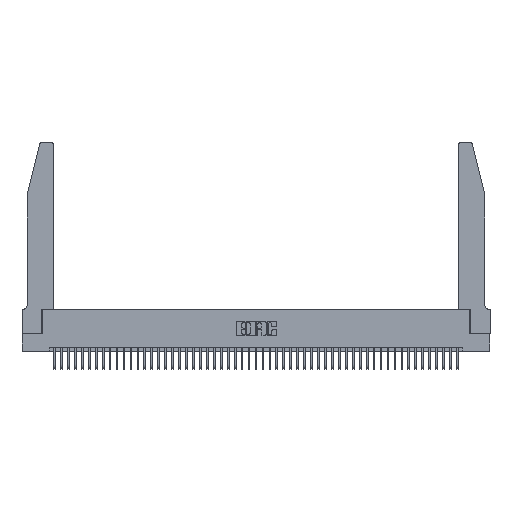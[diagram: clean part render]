
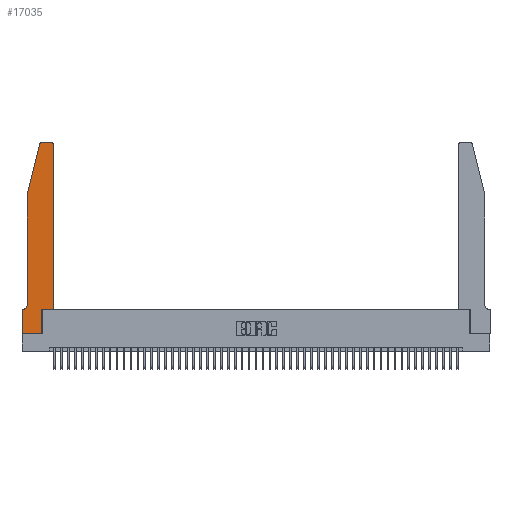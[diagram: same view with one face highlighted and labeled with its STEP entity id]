
A CAD part, top view. The second image highlights one B-rep face of the part: STEP entity #17035.
In plain terms, the highlighted planar face has unit normal (0, 0, 1).
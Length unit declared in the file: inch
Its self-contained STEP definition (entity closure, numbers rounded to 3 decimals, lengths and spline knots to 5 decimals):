
#1237 = AXIS2_PLACEMENT_3D ( 'NONE', #26726, #5091, #30422 ) ;
#1294 = CARTESIAN_POINT ( 'NONE',  ( 0.2865, 0.35, 0.37 ) ) ;
#1839 = FACE_OUTER_BOUND ( 'NONE', #34573, .T. ) ;
#1923 = CARTESIAN_POINT ( 'NONE',  ( 0.4505, 2.72, 0.37 ) ) ;
#2569 = EDGE_CURVE ( 'NONE', #39155, #37777, #5124, .T. ) ;
#3102 = VERTEX_POINT ( 'NONE', #7702 ) ;
#3226 = EDGE_CURVE ( 'NONE', #44333, #39155, #15180, .T. ) ;
#3483 = DIRECTION ( 'NONE',  ( 1., 0., 0. ) ) ;
#3552 = ORIENTED_EDGE ( 'NONE', *, *, #43686, .T. ) ;
#3634 = LINE ( 'NONE', #30653, #21685 ) ;
#3968 = CARTESIAN_POINT ( 'NONE',  ( 0.0755, 2., 0.37 ) ) ;
#4933 = DIRECTION ( 'NONE',  ( 0., 1., 0. ) ) ;
#5091 = DIRECTION ( 'NONE',  ( 0., 0., 1. ) ) ;
#5124 = LINE ( 'NONE', #1294, #23192 ) ;
#5486 = DIRECTION ( 'NONE',  ( 1., 0., 0. ) ) ;
#5744 = CARTESIAN_POINT ( 'NONE',  ( 0.2865, 0.35, 0.37 ) ) ;
#6064 = VERTEX_POINT ( 'NONE', #33162 ) ;
#6067 = VECTOR ( 'NONE', #35936, 39.37008 ) ;
#6370 = VECTOR ( 'NONE', #34168, 39.37008 ) ;
#6822 = VECTOR ( 'NONE', #29985, 39.37008 ) ;
#7702 = CARTESIAN_POINT ( 'NONE',  ( 0.0755, 0.42, 0.37 ) ) ;
#7890 = CARTESIAN_POINT ( 'NONE',  ( 0.284, 2.72, 0.37 ) ) ;
#8151 = LINE ( 'NONE', #14568, #35947 ) ;
#8938 = CIRCLE ( 'NONE', #41493, 0.03 ) ;
#9886 = EDGE_CURVE ( 'NONE', #22141, #3102, #44643, .T. ) ;
#10256 = DIRECTION ( 'NONE',  ( 0., 0., -1. ) ) ;
#11444 = ORIENTED_EDGE ( 'NONE', *, *, #25841, .T. ) ;
#11535 = ORIENTED_EDGE ( 'NONE', *, *, #37563, .T. ) ;
#11543 = DIRECTION ( 'NONE',  ( 1., 0., 0. ) ) ;
#12093 = EDGE_CURVE ( 'NONE', #37777, #46083, #3634, .T. ) ;
#12581 = CARTESIAN_POINT ( 'NONE',  ( 0., 0.35, 0.37 ) ) ;
#14093 = EDGE_CURVE ( 'NONE', #3102, #16471, #29463, .T. ) ;
#14568 = CARTESIAN_POINT ( 'NONE',  ( 0.0755, 2., 0.37 ) ) ;
#14818 = LINE ( 'NONE', #23330, #6370 ) ;
#15180 = LINE ( 'NONE', #41005, #33370 ) ;
#15347 = CARTESIAN_POINT ( 'NONE',  ( 0.4505, 0.35, 0.37 ) ) ;
#15788 = PLANE ( 'NONE',  #1237 ) ;
#16071 = LINE ( 'NONE', #17961, #35427 ) ;
#16227 = VECTOR ( 'NONE', #27158, 39.37008 ) ;
#16444 = VERTEX_POINT ( 'NONE', #30626 ) ;
#16471 = VERTEX_POINT ( 'NONE', #19959 ) ;
#17035 = ADVANCED_FACE ( 'NONE', ( #1839 ), #15788, .T. ) ;
#17961 = CARTESIAN_POINT ( 'NONE',  ( 0.2605, 2.75, 0.37 ) ) ;
#18178 = DIRECTION ( 'NONE',  ( -0.239, -0.971, 0. ) ) ;
#18328 = EDGE_CURVE ( 'NONE', #6064, #42993, #40913, .T. ) ;
#18789 = ORIENTED_EDGE ( 'NONE', *, *, #32397, .T. ) ;
#19389 = ORIENTED_EDGE ( 'NONE', *, *, #2569, .T. ) ;
#19835 = VERTEX_POINT ( 'NONE', #1923 ) ;
#19893 = ORIENTED_EDGE ( 'NONE', *, *, #14093, .T. ) ;
#19959 = CARTESIAN_POINT ( 'NONE',  ( 0.0055, 0.35, 0.37 ) ) ;
#21685 = VECTOR ( 'NONE', #5486, 39.37008 ) ;
#22141 = VERTEX_POINT ( 'NONE', #3968 ) ;
#22804 = CARTESIAN_POINT ( 'NONE',  ( 0.4505, 0.35, 0.37 ) ) ;
#22851 = DIRECTION ( 'NONE',  ( 1., 0., 0. ) ) ;
#23192 = VECTOR ( 'NONE', #4933, 39.37008 ) ;
#23330 = CARTESIAN_POINT ( 'NONE',  ( 0.0755, 0.35, 0.37 ) ) ;
#24068 = EDGE_CURVE ( 'NONE', #19835, #16444, #8938, .T. ) ;
#24372 = ORIENTED_EDGE ( 'NONE', *, *, #35779, .T. ) ;
#25102 = DIRECTION ( 'NONE',  ( 0., 0., 1. ) ) ;
#25841 = EDGE_CURVE ( 'NONE', #16444, #6064, #16071, .T. ) ;
#26061 = LINE ( 'NONE', #15347, #6822 ) ;
#26726 = CARTESIAN_POINT ( 'NONE',  ( 0., 0.35, 0.37 ) ) ;
#27158 = DIRECTION ( 'NONE',  ( 0., -1., 0. ) ) ;
#27617 = AXIS2_PLACEMENT_3D ( 'NONE', #7890, #33242, #11543 ) ;
#28402 = VERTEX_POINT ( 'NONE', #12581 ) ;
#28757 = CARTESIAN_POINT ( 'NONE',  ( 0.0755, 2., 0.37 ) ) ;
#29463 = CIRCLE ( 'NONE', #41853, 0.07 ) ;
#29985 = DIRECTION ( 'NONE',  ( 0., 1., 0. ) ) ;
#30422 = DIRECTION ( 'NONE',  ( 1., 0., 0. ) ) ;
#30626 = CARTESIAN_POINT ( 'NONE',  ( 0.4205, 2.75, 0.37 ) ) ;
#30653 = CARTESIAN_POINT ( 'NONE',  ( 0.4505, 0.35, 0.37 ) ) ;
#31353 = ORIENTED_EDGE ( 'NONE', *, *, #12093, .T. ) ;
#31969 = CARTESIAN_POINT ( 'NONE',  ( 0.0055, 0.42, 0.37 ) ) ;
#32397 = EDGE_CURVE ( 'NONE', #28402, #44333, #44110, .T. ) ;
#33162 = CARTESIAN_POINT ( 'NONE',  ( 0.284, 2.75, 0.37 ) ) ;
#33242 = DIRECTION ( 'NONE',  ( 0., 0., 1. ) ) ;
#33370 = VECTOR ( 'NONE', #22851, 39.37008 ) ;
#33753 = CARTESIAN_POINT ( 'NONE',  ( 0.25487, 2.72718, 0.37 ) ) ;
#34168 = DIRECTION ( 'NONE',  ( -1., 0., 0. ) ) ;
#34358 = CARTESIAN_POINT ( 'NONE',  ( 0., 0., 0.37 ) ) ;
#34573 = EDGE_LOOP ( 'NONE', ( #11444, #39200, #24372, #45470, #19893, #3552, #18789, #35325, #19389, #31353, #11535, #42753 ) ) ;
#35325 = ORIENTED_EDGE ( 'NONE', *, *, #3226, .T. ) ;
#35427 = VECTOR ( 'NONE', #43417, 39.37008 ) ;
#35643 = DIRECTION ( 'NONE',  ( -1., 0., 0. ) ) ;
#35779 = EDGE_CURVE ( 'NONE', #42993, #22141, #8151, .T. ) ;
#35936 = DIRECTION ( 'NONE',  ( 0., -1., 0. ) ) ;
#35947 = VECTOR ( 'NONE', #18178, 39.37008 ) ;
#36103 = CARTESIAN_POINT ( 'NONE',  ( 0.2865, 0., 0.37 ) ) ;
#37563 = EDGE_CURVE ( 'NONE', #46083, #19835, #26061, .T. ) ;
#37777 = VERTEX_POINT ( 'NONE', #5744 ) ;
#39155 = VERTEX_POINT ( 'NONE', #36103 ) ;
#39200 = ORIENTED_EDGE ( 'NONE', *, *, #18328, .T. ) ;
#40913 = CIRCLE ( 'NONE', #27617, 0.03 ) ;
#41005 = CARTESIAN_POINT ( 'NONE',  ( 0., 0., 0.37 ) ) ;
#41493 = AXIS2_PLACEMENT_3D ( 'NONE', #46895, #25102, #3483 ) ;
#41853 = AXIS2_PLACEMENT_3D ( 'NONE', #31969, #10256, #35643 ) ;
#42753 = ORIENTED_EDGE ( 'NONE', *, *, #24068, .T. ) ;
#42993 = VERTEX_POINT ( 'NONE', #33753 ) ;
#43417 = DIRECTION ( 'NONE',  ( -1., 0., 0. ) ) ;
#43686 = EDGE_CURVE ( 'NONE', #16471, #28402, #14818, .T. ) ;
#44110 = LINE ( 'NONE', #34358, #16227 ) ;
#44333 = VERTEX_POINT ( 'NONE', #45376 ) ;
#44643 = LINE ( 'NONE', #28757, #6067 ) ;
#45376 = CARTESIAN_POINT ( 'NONE',  ( 0., 0., 0.37 ) ) ;
#45470 = ORIENTED_EDGE ( 'NONE', *, *, #9886, .T. ) ;
#46083 = VERTEX_POINT ( 'NONE', #22804 ) ;
#46895 = CARTESIAN_POINT ( 'NONE',  ( 0.4205, 2.72, 0.37 ) ) ;
